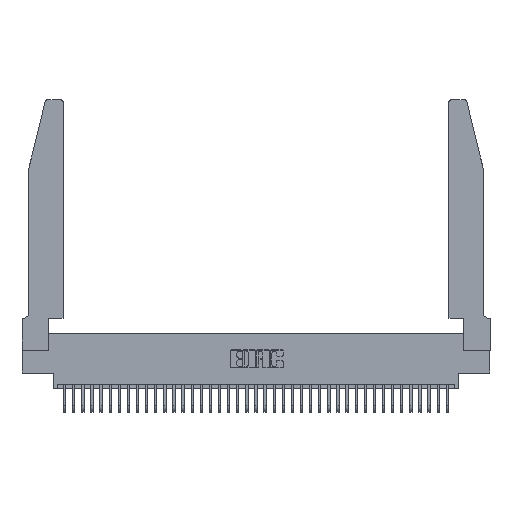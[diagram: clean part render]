
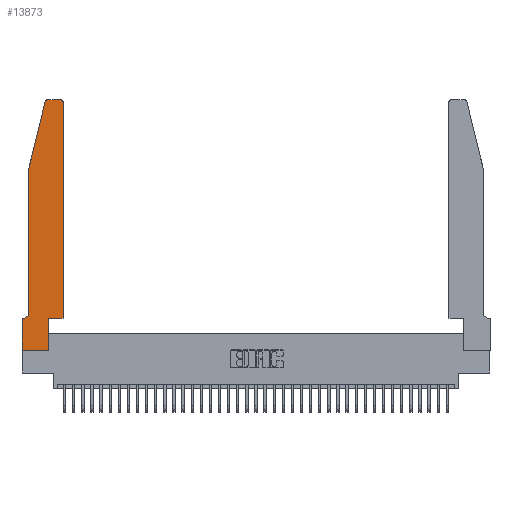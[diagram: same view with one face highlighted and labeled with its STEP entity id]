
A CAD part, top view. The second image highlights one B-rep face of the part: STEP entity #13873.
In plain terms, the highlighted planar face has unit normal (0, 0, 1).
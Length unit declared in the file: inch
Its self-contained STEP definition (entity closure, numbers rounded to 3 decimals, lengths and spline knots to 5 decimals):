
#179 = VECTOR ( 'NONE', #24142, 39.37008 ) ;
#636 = DIRECTION ( 'NONE',  ( 1., 0., 0. ) ) ;
#639 = EDGE_CURVE ( 'NONE', #39201, #14887, #7011, .T. ) ;
#688 = CARTESIAN_POINT ( 'NONE',  ( 0.0755, 2., 0.37 ) ) ;
#790 = VECTOR ( 'NONE', #5918, 39.37008 ) ;
#1221 = CIRCLE ( 'NONE', #28188, 0.03 ) ;
#1609 = VERTEX_POINT ( 'NONE', #27325 ) ;
#2048 = DIRECTION ( 'NONE',  ( 1., 0., 0. ) ) ;
#2095 = VERTEX_POINT ( 'NONE', #37796 ) ;
#2488 = VECTOR ( 'NONE', #26967, 39.37008 ) ;
#2529 = VERTEX_POINT ( 'NONE', #33506 ) ;
#3427 = ORIENTED_EDGE ( 'NONE', *, *, #26739, .T. ) ;
#3553 = EDGE_CURVE ( 'NONE', #16518, #20759, #10230, .T. ) ;
#4158 = EDGE_CURVE ( 'NONE', #20759, #39201, #37841, .T. ) ;
#5918 = DIRECTION ( 'NONE',  ( -1., 0., 0. ) ) ;
#6298 = ORIENTED_EDGE ( 'NONE', *, *, #639, .T. ) ;
#7011 = LINE ( 'NONE', #14618, #13833 ) ;
#7816 = EDGE_CURVE ( 'NONE', #12421, #18884, #1221, .T. ) ;
#8010 = DIRECTION ( 'NONE',  ( 0., -1., 0. ) ) ;
#8033 = CARTESIAN_POINT ( 'NONE',  ( 0.4205, 2.72, 0.37 ) ) ;
#8066 = LINE ( 'NONE', #27536, #19206 ) ;
#8118 = ORIENTED_EDGE ( 'NONE', *, *, #4158, .T. ) ;
#8162 = VECTOR ( 'NONE', #38794, 39.37008 ) ;
#8832 = ORIENTED_EDGE ( 'NONE', *, *, #24011, .T. ) ;
#9943 = CIRCLE ( 'NONE', #12018, 0.03 ) ;
#10003 = EDGE_CURVE ( 'NONE', #18884, #2529, #15158, .T. ) ;
#10230 = LINE ( 'NONE', #33393, #2488 ) ;
#10482 = VERTEX_POINT ( 'NONE', #34230 ) ;
#10973 = DIRECTION ( 'NONE',  ( 0., 0., 1. ) ) ;
#11833 = AXIS2_PLACEMENT_3D ( 'NONE', #31896, #14377, #2048 ) ;
#12018 = AXIS2_PLACEMENT_3D ( 'NONE', #8033, #32163, #14402 ) ;
#12421 = VERTEX_POINT ( 'NONE', #26673 ) ;
#13018 = CARTESIAN_POINT ( 'NONE',  ( 0.0055, 0.42, 0.37 ) ) ;
#13833 = VECTOR ( 'NONE', #636, 39.37008 ) ;
#13873 = ADVANCED_FACE ( 'NONE', ( #28829 ), #35533, .T. ) ;
#13984 = CARTESIAN_POINT ( 'NONE',  ( 0.4505, 0.35, 0.37 ) ) ;
#14195 = DIRECTION ( 'NONE',  ( 1., 0., 0. ) ) ;
#14377 = DIRECTION ( 'NONE',  ( 0., 0., 1. ) ) ;
#14379 = CARTESIAN_POINT ( 'NONE',  ( 0., 0., 0.37 ) ) ;
#14402 = DIRECTION ( 'NONE',  ( 1., 0., 0. ) ) ;
#14618 = CARTESIAN_POINT ( 'NONE',  ( 0., 0., 0.37 ) ) ;
#14887 = VERTEX_POINT ( 'NONE', #35071 ) ;
#15158 = LINE ( 'NONE', #688, #16092 ) ;
#16049 = DIRECTION ( 'NONE',  ( 1., 0., 0. ) ) ;
#16092 = VECTOR ( 'NONE', #32306, 39.37008 ) ;
#16128 = CARTESIAN_POINT ( 'NONE',  ( 0.4205, 2.75, 0.37 ) ) ;
#16404 = DIRECTION ( 'NONE',  ( -1., 0., 0. ) ) ;
#16518 = VERTEX_POINT ( 'NONE', #33108 ) ;
#17541 = ORIENTED_EDGE ( 'NONE', *, *, #28001, .T. ) ;
#17886 = CARTESIAN_POINT ( 'NONE',  ( 0.4505, 0.35, 0.37 ) ) ;
#18084 = CARTESIAN_POINT ( 'NONE',  ( 0.0755, 2., 0.37 ) ) ;
#18313 = LINE ( 'NONE', #25290, #790 ) ;
#18813 = LINE ( 'NONE', #13984, #8162 ) ;
#18819 = CARTESIAN_POINT ( 'NONE',  ( 0.25487, 2.72718, 0.37 ) ) ;
#18884 = VERTEX_POINT ( 'NONE', #18819 ) ;
#19206 = VECTOR ( 'NONE', #16049, 39.37008 ) ;
#19805 = EDGE_CURVE ( 'NONE', #10482, #23895, #8066, .T. ) ;
#20245 = CARTESIAN_POINT ( 'NONE',  ( 0., 0.35, 0.37 ) ) ;
#20393 = ORIENTED_EDGE ( 'NONE', *, *, #7816, .T. ) ;
#20759 = VERTEX_POINT ( 'NONE', #20245 ) ;
#22301 = DIRECTION ( 'NONE',  ( 0., 0., -1. ) ) ;
#22386 = ORIENTED_EDGE ( 'NONE', *, *, #19805, .T. ) ;
#23895 = VERTEX_POINT ( 'NONE', #17886 ) ;
#24011 = EDGE_CURVE ( 'NONE', #32676, #12421, #18313, .T. ) ;
#24142 = DIRECTION ( 'NONE',  ( 0., -1., 0. ) ) ;
#24382 = ORIENTED_EDGE ( 'NONE', *, *, #3553, .T. ) ;
#25290 = CARTESIAN_POINT ( 'NONE',  ( 0.2605, 2.75, 0.37 ) ) ;
#26307 = ORIENTED_EDGE ( 'NONE', *, *, #37071, .T. ) ;
#26673 = CARTESIAN_POINT ( 'NONE',  ( 0.284, 2.75, 0.37 ) ) ;
#26739 = EDGE_CURVE ( 'NONE', #1609, #16518, #35740, .T. ) ;
#26950 = ORIENTED_EDGE ( 'NONE', *, *, #34074, .T. ) ;
#26967 = DIRECTION ( 'NONE',  ( -1., 0., 0. ) ) ;
#27197 = CARTESIAN_POINT ( 'NONE',  ( 0.2865, 0.35, 0.37 ) ) ;
#27325 = CARTESIAN_POINT ( 'NONE',  ( 0.0755, 0.42, 0.37 ) ) ;
#27473 = DIRECTION ( 'NONE',  ( 0., 1., 0. ) ) ;
#27536 = CARTESIAN_POINT ( 'NONE',  ( 0.4505, 0.35, 0.37 ) ) ;
#27853 = CARTESIAN_POINT ( 'NONE',  ( 0., 0., 0.37 ) ) ;
#28001 = EDGE_CURVE ( 'NONE', #2529, #1609, #33676, .T. ) ;
#28188 = AXIS2_PLACEMENT_3D ( 'NONE', #29508, #10973, #14195 ) ;
#28829 = FACE_OUTER_BOUND ( 'NONE', #38019, .T. ) ;
#29508 = CARTESIAN_POINT ( 'NONE',  ( 0.284, 2.72, 0.37 ) ) ;
#30617 = LINE ( 'NONE', #27197, #32073 ) ;
#31896 = CARTESIAN_POINT ( 'NONE',  ( 0., 0.35, 0.37 ) ) ;
#32073 = VECTOR ( 'NONE', #27473, 39.37008 ) ;
#32122 = EDGE_CURVE ( 'NONE', #23895, #2095, #18813, .T. ) ;
#32163 = DIRECTION ( 'NONE',  ( 0., 0., 1. ) ) ;
#32306 = DIRECTION ( 'NONE',  ( -0.239, -0.971, 0. ) ) ;
#32676 = VERTEX_POINT ( 'NONE', #16128 ) ;
#33108 = CARTESIAN_POINT ( 'NONE',  ( 0.0055, 0.35, 0.37 ) ) ;
#33393 = CARTESIAN_POINT ( 'NONE',  ( 0.0755, 0.35, 0.37 ) ) ;
#33506 = CARTESIAN_POINT ( 'NONE',  ( 0.0755, 2., 0.37 ) ) ;
#33540 = ORIENTED_EDGE ( 'NONE', *, *, #10003, .T. ) ;
#33676 = LINE ( 'NONE', #18084, #179 ) ;
#34074 = EDGE_CURVE ( 'NONE', #2095, #32676, #9943, .T. ) ;
#34230 = CARTESIAN_POINT ( 'NONE',  ( 0.2865, 0.35, 0.37 ) ) ;
#35071 = CARTESIAN_POINT ( 'NONE',  ( 0.2865, 0., 0.37 ) ) ;
#35533 = PLANE ( 'NONE',  #11833 ) ;
#35740 = CIRCLE ( 'NONE', #37064, 0.07 ) ;
#37064 = AXIS2_PLACEMENT_3D ( 'NONE', #13018, #22301, #16404 ) ;
#37071 = EDGE_CURVE ( 'NONE', #14887, #10482, #30617, .T. ) ;
#37796 = CARTESIAN_POINT ( 'NONE',  ( 0.4505, 2.72, 0.37 ) ) ;
#37841 = LINE ( 'NONE', #14379, #38359 ) ;
#38019 = EDGE_LOOP ( 'NONE', ( #8832, #20393, #33540, #17541, #3427, #24382, #8118, #6298, #26307, #22386, #39377, #26950 ) ) ;
#38359 = VECTOR ( 'NONE', #8010, 39.37008 ) ;
#38794 = DIRECTION ( 'NONE',  ( 0., 1., 0. ) ) ;
#39201 = VERTEX_POINT ( 'NONE', #27853 ) ;
#39377 = ORIENTED_EDGE ( 'NONE', *, *, #32122, .T. ) ;
